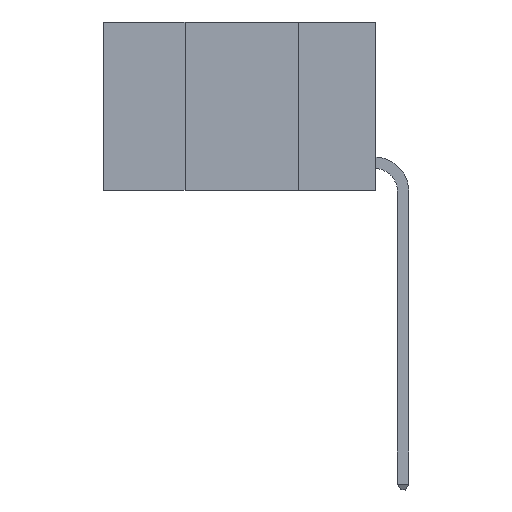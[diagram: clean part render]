
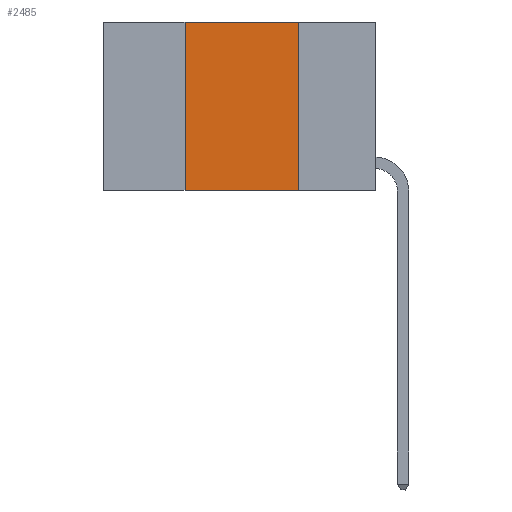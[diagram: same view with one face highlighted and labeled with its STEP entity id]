
A CAD part, left-side view. The second image highlights one B-rep face of the part: STEP entity #2485.
In plain terms, the highlighted planar face has unit normal (-1, 0, 0).
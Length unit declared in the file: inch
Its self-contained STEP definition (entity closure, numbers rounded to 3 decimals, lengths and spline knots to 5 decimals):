
#987 = CARTESIAN_POINT ( 'NONE',  ( 0., 0.17, -0.37 ) ) ;
#1055 = VECTOR ( 'NONE', #12782, 39.37008 ) ;
#1825 = VECTOR ( 'NONE', #15716, 39.37008 ) ;
#1871 = ORIENTED_EDGE ( 'NONE', *, *, #16957, .F. ) ;
#2351 = CARTESIAN_POINT ( 'NONE',  ( 0., 0.6, 0. ) ) ;
#2485 = ADVANCED_FACE ( 'NONE', ( #9381 ), #16547, .F. ) ;
#2512 = CARTESIAN_POINT ( 'NONE',  ( 0., 0.17, 0. ) ) ;
#2572 = DIRECTION ( 'NONE',  ( 1., 0., 0. ) ) ;
#3241 = VERTEX_POINT ( 'NONE', #987 ) ;
#3839 = CARTESIAN_POINT ( 'NONE',  ( 0., 0.17, 0. ) ) ;
#5524 = CARTESIAN_POINT ( 'NONE',  ( 0., 0.42, 0. ) ) ;
#5633 = AXIS2_PLACEMENT_3D ( 'NONE', #7237, #2572, #13992 ) ;
#6067 = VECTOR ( 'NONE', #10739, 39.37008 ) ;
#6279 = CARTESIAN_POINT ( 'NONE',  ( 0., 0.6, -0.37 ) ) ;
#6285 = EDGE_CURVE ( 'NONE', #12308, #12933, #16169, .T. ) ;
#7237 = CARTESIAN_POINT ( 'NONE',  ( 0., 0.6, 0. ) ) ;
#8499 = EDGE_CURVE ( 'NONE', #12933, #3241, #12911, .T. ) ;
#9381 = FACE_OUTER_BOUND ( 'NONE', #9620, .T. ) ;
#9620 = EDGE_LOOP ( 'NONE', ( #17102, #14559, #1871, #10670 ) ) ;
#10670 = ORIENTED_EDGE ( 'NONE', *, *, #11975, .T. ) ;
#10739 = DIRECTION ( 'NONE',  ( 0., -1., 0. ) ) ;
#11325 = CARTESIAN_POINT ( 'NONE',  ( 0., 0.42, 0. ) ) ;
#11850 = CARTESIAN_POINT ( 'NONE',  ( 0., 0.42, -0.37 ) ) ;
#11975 = EDGE_CURVE ( 'NONE', #13142, #3241, #17704, .T. ) ;
#12308 = VERTEX_POINT ( 'NONE', #5524 ) ;
#12316 = VECTOR ( 'NONE', #14210, 39.37008 ) ;
#12782 = DIRECTION ( 'NONE',  ( 0., 0., -1. ) ) ;
#12911 = LINE ( 'NONE', #3839, #1055 ) ;
#12933 = VERTEX_POINT ( 'NONE', #2512 ) ;
#13142 = VERTEX_POINT ( 'NONE', #11850 ) ;
#13992 = DIRECTION ( 'NONE',  ( 0., 0., -1. ) ) ;
#14210 = DIRECTION ( 'NONE',  ( 0., -1., 0. ) ) ;
#14559 = ORIENTED_EDGE ( 'NONE', *, *, #6285, .F. ) ;
#15716 = DIRECTION ( 'NONE',  ( 0., 0., 1. ) ) ;
#16169 = LINE ( 'NONE', #2351, #12316 ) ;
#16547 = PLANE ( 'NONE',  #5633 ) ;
#16608 = LINE ( 'NONE', #11325, #1825 ) ;
#16957 = EDGE_CURVE ( 'NONE', #13142, #12308, #16608, .T. ) ;
#17102 = ORIENTED_EDGE ( 'NONE', *, *, #8499, .F. ) ;
#17704 = LINE ( 'NONE', #6279, #6067 ) ;
